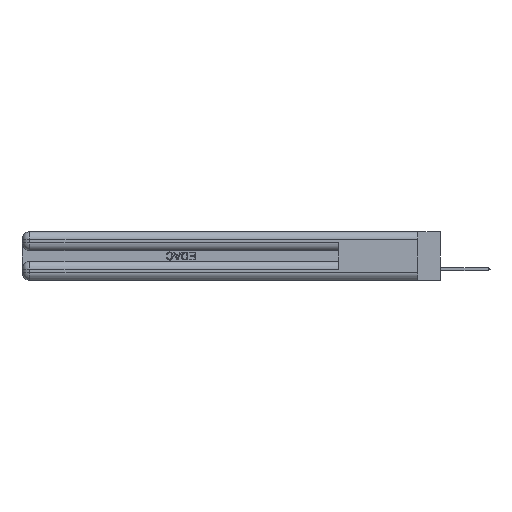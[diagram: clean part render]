
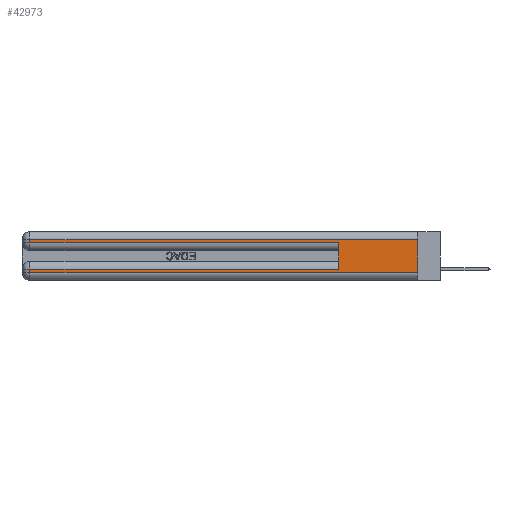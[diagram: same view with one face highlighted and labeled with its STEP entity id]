
A CAD part, left-side view. The second image highlights one B-rep face of the part: STEP entity #42973.
In plain terms, the highlighted planar face has unit normal (-1, 0, 0).
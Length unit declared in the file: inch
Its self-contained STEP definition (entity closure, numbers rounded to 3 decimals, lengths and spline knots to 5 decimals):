
#1694 = EDGE_CURVE ( 'NONE', #12275, #38060, #44489, .T. ) ;
#2942 = CARTESIAN_POINT ( 'NONE',  ( 0., 2.94, 0.06 ) ) ;
#3622 = ORIENTED_EDGE ( 'NONE', *, *, #15620, .T. ) ;
#3657 = CARTESIAN_POINT ( 'NONE',  ( 0., 0., 0.37 ) ) ;
#3855 = CARTESIAN_POINT ( 'NONE',  ( 0., 0., 0.085 ) ) ;
#3935 = DIRECTION ( 'NONE',  ( 0., -1., 0. ) ) ;
#4758 = DIRECTION ( 'NONE',  ( 0., 0., -1. ) ) ;
#5074 = DIRECTION ( 'NONE',  ( 1., 0., 0. ) ) ;
#5502 = DIRECTION ( 'NONE',  ( 0., 0., 1. ) ) ;
#5690 = DIRECTION ( 'NONE',  ( 0., -1., 0. ) ) ;
#5932 = EDGE_CURVE ( 'NONE', #14627, #41945, #15733, .T. ) ;
#6370 = VECTOR ( 'NONE', #25846, 39.37008 ) ;
#6664 = ORIENTED_EDGE ( 'NONE', *, *, #21711, .F. ) ;
#6725 = CARTESIAN_POINT ( 'NONE',  ( 0., 0.6, 0.285 ) ) ;
#7309 = CARTESIAN_POINT ( 'NONE',  ( 0., 0., 0.285 ) ) ;
#7612 = VECTOR ( 'NONE', #5690, 39.37008 ) ;
#9265 = CARTESIAN_POINT ( 'NONE',  ( 0., 0., 0.31 ) ) ;
#9536 = VERTEX_POINT ( 'NONE', #6725 ) ;
#9611 = CARTESIAN_POINT ( 'NONE',  ( 0., 2.94, 0.085 ) ) ;
#11617 = VECTOR ( 'NONE', #5502, 39.37008 ) ;
#11697 = VECTOR ( 'NONE', #13357, 39.37008 ) ;
#12275 = VERTEX_POINT ( 'NONE', #34117 ) ;
#12328 = CARTESIAN_POINT ( 'NONE',  ( 0., 2.94, 0.37 ) ) ;
#13357 = DIRECTION ( 'NONE',  ( 0., 0., -1. ) ) ;
#13670 = LINE ( 'NONE', #7309, #17557 ) ;
#14000 = ORIENTED_EDGE ( 'NONE', *, *, #24241, .T. ) ;
#14454 = CARTESIAN_POINT ( 'NONE',  ( 0., 2.94, 0.37 ) ) ;
#14593 = VECTOR ( 'NONE', #45623, 39.37008 ) ;
#14627 = VERTEX_POINT ( 'NONE', #9265 ) ;
#14967 = CARTESIAN_POINT ( 'NONE',  ( 0., 0., 0.06 ) ) ;
#15620 = EDGE_CURVE ( 'NONE', #15791, #33945, #17563, .T. ) ;
#15733 = LINE ( 'NONE', #25247, #6370 ) ;
#15791 = VERTEX_POINT ( 'NONE', #2942 ) ;
#15871 = PLANE ( 'NONE',  #36001 ) ;
#16455 = ORIENTED_EDGE ( 'NONE', *, *, #5932, .T. ) ;
#17557 = VECTOR ( 'NONE', #3935, 39.37008 ) ;
#17563 = LINE ( 'NONE', #14967, #7612 ) ;
#19430 = CARTESIAN_POINT ( 'NONE',  ( 0., 0., 0.37 ) ) ;
#21355 = FACE_OUTER_BOUND ( 'NONE', #38611, .T. ) ;
#21407 = ORIENTED_EDGE ( 'NONE', *, *, #44580, .F. ) ;
#21711 = EDGE_CURVE ( 'NONE', #12275, #9536, #32583, .T. ) ;
#21880 = VERTEX_POINT ( 'NONE', #25580 ) ;
#23019 = ORIENTED_EDGE ( 'NONE', *, *, #44235, .T. ) ;
#24241 = EDGE_CURVE ( 'NONE', #21880, #9536, #13670, .T. ) ;
#25126 = LINE ( 'NONE', #3657, #14593 ) ;
#25247 = CARTESIAN_POINT ( 'NONE',  ( 0., 0., 0.31 ) ) ;
#25580 = CARTESIAN_POINT ( 'NONE',  ( 0., 2.94, 0.285 ) ) ;
#25754 = VECTOR ( 'NONE', #34411, 39.37008 ) ;
#25846 = DIRECTION ( 'NONE',  ( 0., 1., 0. ) ) ;
#26627 = CARTESIAN_POINT ( 'NONE',  ( 0., 0.6, 0.145 ) ) ;
#28429 = ORIENTED_EDGE ( 'NONE', *, *, #37266, .T. ) ;
#32583 = LINE ( 'NONE', #26627, #11617 ) ;
#33945 = VERTEX_POINT ( 'NONE', #42412 ) ;
#34117 = CARTESIAN_POINT ( 'NONE',  ( 0., 0.6, 0.085 ) ) ;
#34411 = DIRECTION ( 'NONE',  ( 0., 1., 0. ) ) ;
#34431 = CARTESIAN_POINT ( 'NONE',  ( 0., 2.94, 0.31 ) ) ;
#35361 = LINE ( 'NONE', #14454, #11697 ) ;
#36001 = AXIS2_PLACEMENT_3D ( 'NONE', #19430, #5074, #4758 ) ;
#36121 = LINE ( 'NONE', #12328, #37296 ) ;
#37266 = EDGE_CURVE ( 'NONE', #41945, #21880, #35361, .T. ) ;
#37296 = VECTOR ( 'NONE', #44196, 39.37008 ) ;
#38060 = VERTEX_POINT ( 'NONE', #9611 ) ;
#38611 = EDGE_LOOP ( 'NONE', ( #21407, #16455, #28429, #14000, #6664, #45154, #23019, #3622 ) ) ;
#41945 = VERTEX_POINT ( 'NONE', #34431 ) ;
#42412 = CARTESIAN_POINT ( 'NONE',  ( 0., 0., 0.06 ) ) ;
#42973 = ADVANCED_FACE ( 'NONE', ( #21355 ), #15871, .F. ) ;
#44196 = DIRECTION ( 'NONE',  ( 0., 0., -1. ) ) ;
#44235 = EDGE_CURVE ( 'NONE', #38060, #15791, #36121, .T. ) ;
#44489 = LINE ( 'NONE', #3855, #25754 ) ;
#44580 = EDGE_CURVE ( 'NONE', #14627, #33945, #25126, .T. ) ;
#45154 = ORIENTED_EDGE ( 'NONE', *, *, #1694, .T. ) ;
#45623 = DIRECTION ( 'NONE',  ( 0., 0., -1. ) ) ;
